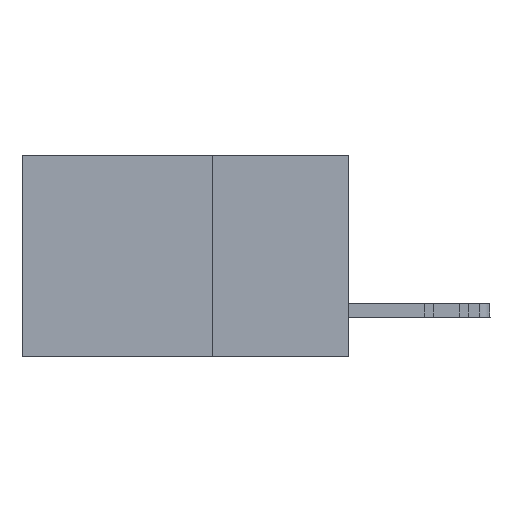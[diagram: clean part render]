
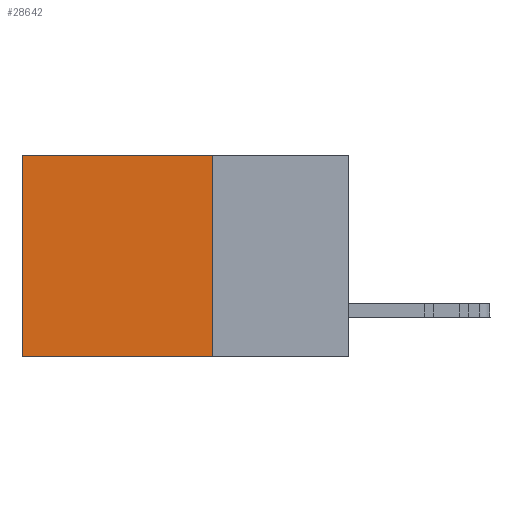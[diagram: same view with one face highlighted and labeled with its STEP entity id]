
A CAD part, left-side view. The second image highlights one B-rep face of the part: STEP entity #28642.
In plain terms, the highlighted planar face has unit normal (-1, 0, 0).
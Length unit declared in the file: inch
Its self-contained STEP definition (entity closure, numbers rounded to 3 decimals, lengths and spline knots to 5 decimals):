
#339 = DIRECTION ( 'NONE',  ( 1., 0., 0. ) ) ;
#497 = CARTESIAN_POINT ( 'NONE',  ( 0.298, 0.25, -0.37 ) ) ;
#1087 = ORIENTED_EDGE ( 'NONE', *, *, #17107, .F. ) ;
#1677 = CARTESIAN_POINT ( 'NONE',  ( 0.298, 0.25, 0. ) ) ;
#2812 = CARTESIAN_POINT ( 'NONE',  ( 0.298, 0.25, 0. ) ) ;
#3170 = CARTESIAN_POINT ( 'NONE',  ( 0.298, 0.6, 0. ) ) ;
#4712 = EDGE_CURVE ( 'NONE', #12358, #17990, #26340, .T. ) ;
#5443 = DIRECTION ( 'NONE',  ( 0., 0., -1. ) ) ;
#5718 = CARTESIAN_POINT ( 'NONE',  ( 0.298, 0.6, 0. ) ) ;
#6628 = CARTESIAN_POINT ( 'NONE',  ( 0.298, 0.25, 0. ) ) ;
#6731 = DIRECTION ( 'NONE',  ( 0., 1., 0. ) ) ;
#9214 = ORIENTED_EDGE ( 'NONE', *, *, #19685, .T. ) ;
#9750 = PLANE ( 'NONE',  #13415 ) ;
#9941 = DIRECTION ( 'NONE',  ( 0., 0., -1. ) ) ;
#10358 = FACE_OUTER_BOUND ( 'NONE', #16863, .T. ) ;
#10655 = CARTESIAN_POINT ( 'NONE',  ( 0.298, 0.25, -0.37 ) ) ;
#11923 = LINE ( 'NONE', #14274, #26600 ) ;
#12290 = ORIENTED_EDGE ( 'NONE', *, *, #4712, .T. ) ;
#12358 = VERTEX_POINT ( 'NONE', #5718 ) ;
#13220 = DIRECTION ( 'NONE',  ( 0., 0., -1. ) ) ;
#13415 = AXIS2_PLACEMENT_3D ( 'NONE', #2812, #339, #9941 ) ;
#14274 = CARTESIAN_POINT ( 'NONE',  ( 0.298, 0.25, 0. ) ) ;
#15916 = VECTOR ( 'NONE', #6731, 39.37008 ) ;
#16863 = EDGE_LOOP ( 'NONE', ( #12290, #1087, #20104, #9214 ) ) ;
#17107 = EDGE_CURVE ( 'NONE', #23961, #17990, #18171, .T. ) ;
#17990 = VERTEX_POINT ( 'NONE', #20837 ) ;
#18171 = LINE ( 'NONE', #10655, #19641 ) ;
#19641 = VECTOR ( 'NONE', #22252, 39.37008 ) ;
#19685 = EDGE_CURVE ( 'NONE', #22961, #12358, #30269, .T. ) ;
#20104 = ORIENTED_EDGE ( 'NONE', *, *, #21890, .F. ) ;
#20837 = CARTESIAN_POINT ( 'NONE',  ( 0.298, 0.6, -0.37 ) ) ;
#21890 = EDGE_CURVE ( 'NONE', #22961, #23961, #11923, .T. ) ;
#22252 = DIRECTION ( 'NONE',  ( 0., 1., 0. ) ) ;
#22645 = VECTOR ( 'NONE', #13220, 39.37008 ) ;
#22961 = VERTEX_POINT ( 'NONE', #1677 ) ;
#23961 = VERTEX_POINT ( 'NONE', #497 ) ;
#26340 = LINE ( 'NONE', #3170, #22645 ) ;
#26600 = VECTOR ( 'NONE', #5443, 39.37008 ) ;
#28642 = ADVANCED_FACE ( 'NONE', ( #10358 ), #9750, .F. ) ;
#30269 = LINE ( 'NONE', #6628, #15916 ) ;
